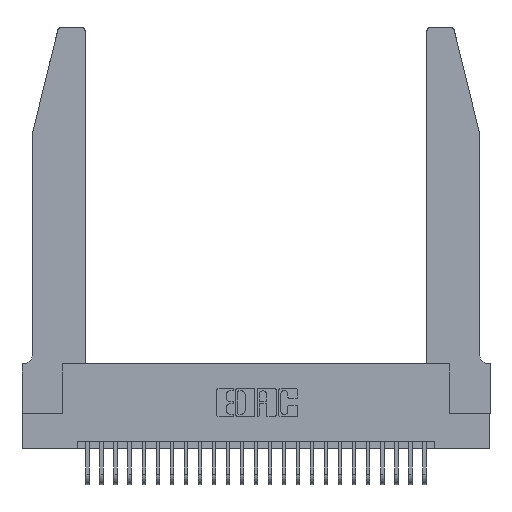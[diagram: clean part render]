
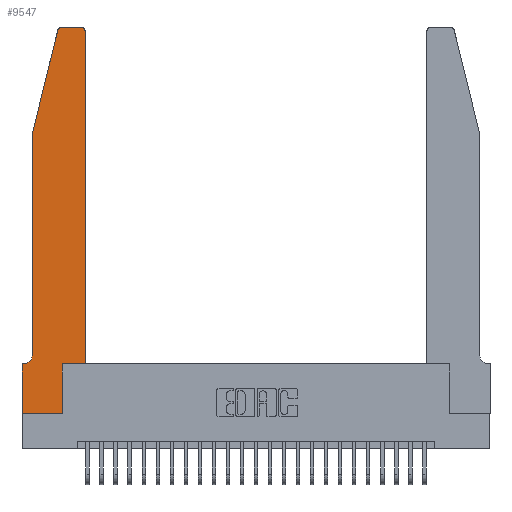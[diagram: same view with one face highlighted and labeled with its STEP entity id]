
A CAD part, top view. The second image highlights one B-rep face of the part: STEP entity #9547.
In plain terms, the highlighted planar face has unit normal (0, 0, 1).
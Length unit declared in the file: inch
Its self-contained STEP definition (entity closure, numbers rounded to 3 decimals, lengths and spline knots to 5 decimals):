
#465 = LINE ( 'NONE', #25406, #22419 ) ;
#1159 = PLANE ( 'NONE',  #19216 ) ;
#1476 = VECTOR ( 'NONE', #2208, 39.37008 ) ;
#1541 = CIRCLE ( 'NONE', #20087, 0.07 ) ;
#1642 = VERTEX_POINT ( 'NONE', #18377 ) ;
#1808 = CARTESIAN_POINT ( 'NONE',  ( 0.4505, 0.35, 0.37 ) ) ;
#1850 = ORIENTED_EDGE ( 'NONE', *, *, #24997, .T. ) ;
#2022 = EDGE_CURVE ( 'NONE', #19401, #26166, #21183, .T. ) ;
#2190 = CARTESIAN_POINT ( 'NONE',  ( 0.0755, 2., 0.37 ) ) ;
#2208 = DIRECTION ( 'NONE',  ( 0., -1., 0. ) ) ;
#2217 = EDGE_LOOP ( 'NONE', ( #2348, #25640, #6581, #22094, #24054, #10860, #9317, #10943, #26642, #17401, #20785, #1850 ) ) ;
#2271 = EDGE_CURVE ( 'NONE', #21834, #15559, #9877, .T. ) ;
#2348 = ORIENTED_EDGE ( 'NONE', *, *, #2634, .T. ) ;
#2413 = CARTESIAN_POINT ( 'NONE',  ( 0.25487, 2.72718, 0.37 ) ) ;
#2634 = EDGE_CURVE ( 'NONE', #8302, #1642, #24844, .T. ) ;
#2862 = CARTESIAN_POINT ( 'NONE',  ( 0.4205, 2.75, 0.37 ) ) ;
#2946 = CARTESIAN_POINT ( 'NONE',  ( 0.0055, 0.35, 0.37 ) ) ;
#3016 = VERTEX_POINT ( 'NONE', #5302 ) ;
#3129 = CARTESIAN_POINT ( 'NONE',  ( 0.4205, 2.72, 0.37 ) ) ;
#3370 = DIRECTION ( 'NONE',  ( 1., 0., 0. ) ) ;
#4426 = DIRECTION ( 'NONE',  ( -0.239, -0.971, 0. ) ) ;
#5302 = CARTESIAN_POINT ( 'NONE',  ( 0.4505, 2.72, 0.37 ) ) ;
#5370 = DIRECTION ( 'NONE',  ( 1., 0., 0. ) ) ;
#5846 = AXIS2_PLACEMENT_3D ( 'NONE', #11664, #26848, #13917 ) ;
#6477 = LINE ( 'NONE', #13195, #23227 ) ;
#6581 = ORIENTED_EDGE ( 'NONE', *, *, #9818, .T. ) ;
#6863 = VERTEX_POINT ( 'NONE', #2413 ) ;
#7178 = CARTESIAN_POINT ( 'NONE',  ( 0.0755, 2., 0.37 ) ) ;
#7501 = VECTOR ( 'NONE', #8138, 39.37008 ) ;
#8138 = DIRECTION ( 'NONE',  ( 1., 0., 0. ) ) ;
#8302 = VERTEX_POINT ( 'NONE', #2862 ) ;
#8848 = VECTOR ( 'NONE', #10862, 39.37008 ) ;
#8885 = DIRECTION ( 'NONE',  ( -1., 0., 0. ) ) ;
#9123 = CARTESIAN_POINT ( 'NONE',  ( 0.0055, 0.42, 0.37 ) ) ;
#9317 = ORIENTED_EDGE ( 'NONE', *, *, #11057, .T. ) ;
#9547 = ADVANCED_FACE ( 'NONE', ( #15391 ), #1159, .T. ) ;
#9818 = EDGE_CURVE ( 'NONE', #6863, #21834, #20143, .T. ) ;
#9849 = CARTESIAN_POINT ( 'NONE',  ( 0.2865, 0.35, 0.37 ) ) ;
#9877 = LINE ( 'NONE', #7178, #25870 ) ;
#10860 = ORIENTED_EDGE ( 'NONE', *, *, #11080, .T. ) ;
#10862 = DIRECTION ( 'NONE',  ( 0., 1., 0. ) ) ;
#10899 = CARTESIAN_POINT ( 'NONE',  ( 0.0755, 2., 0.37 ) ) ;
#10943 = ORIENTED_EDGE ( 'NONE', *, *, #13175, .T. ) ;
#11057 = EDGE_CURVE ( 'NONE', #18265, #21191, #13936, .T. ) ;
#11080 = EDGE_CURVE ( 'NONE', #24962, #18265, #19053, .T. ) ;
#11344 = DIRECTION ( 'NONE',  ( -1., 0., 0. ) ) ;
#11621 = VERTEX_POINT ( 'NONE', #1808 ) ;
#11664 = CARTESIAN_POINT ( 'NONE',  ( 0.284, 2.72, 0.37 ) ) ;
#12181 = CARTESIAN_POINT ( 'NONE',  ( 0., 0.35, 0.37 ) ) ;
#12538 = VECTOR ( 'NONE', #8885, 39.37008 ) ;
#13175 = EDGE_CURVE ( 'NONE', #21191, #19401, #465, .T. ) ;
#13195 = CARTESIAN_POINT ( 'NONE',  ( 0.4505, 0.35, 0.37 ) ) ;
#13917 = DIRECTION ( 'NONE',  ( 1., 0., 0. ) ) ;
#13936 = LINE ( 'NONE', #19848, #1476 ) ;
#14284 = AXIS2_PLACEMENT_3D ( 'NONE', #3129, #18554, #5370 ) ;
#14348 = VECTOR ( 'NONE', #4426, 39.37008 ) ;
#15391 = FACE_OUTER_BOUND ( 'NONE', #2217, .T. ) ;
#15410 = DIRECTION ( 'NONE',  ( 0., 1., 0. ) ) ;
#15559 = VERTEX_POINT ( 'NONE', #16978 ) ;
#16593 = DIRECTION ( 'NONE',  ( 0., 0., 1. ) ) ;
#16822 = DIRECTION ( 'NONE',  ( 1., 0., 0. ) ) ;
#16978 = CARTESIAN_POINT ( 'NONE',  ( 0.0755, 0.42, 0.37 ) ) ;
#17401 = ORIENTED_EDGE ( 'NONE', *, *, #17478, .T. ) ;
#17478 = EDGE_CURVE ( 'NONE', #26166, #11621, #22882, .T. ) ;
#17486 = CARTESIAN_POINT ( 'NONE',  ( 0.2865, 0.35, 0.37 ) ) ;
#17915 = CIRCLE ( 'NONE', #5846, 0.03 ) ;
#18265 = VERTEX_POINT ( 'NONE', #25916 ) ;
#18377 = CARTESIAN_POINT ( 'NONE',  ( 0.284, 2.75, 0.37 ) ) ;
#18554 = DIRECTION ( 'NONE',  ( 0., 0., 1. ) ) ;
#19053 = LINE ( 'NONE', #21982, #12538 ) ;
#19216 = AXIS2_PLACEMENT_3D ( 'NONE', #12181, #16593, #3370 ) ;
#19279 = CARTESIAN_POINT ( 'NONE',  ( 0.2605, 2.75, 0.37 ) ) ;
#19401 = VERTEX_POINT ( 'NONE', #27067 ) ;
#19848 = CARTESIAN_POINT ( 'NONE',  ( 0., 0., 0.37 ) ) ;
#19919 = EDGE_CURVE ( 'NONE', #1642, #6863, #17915, .T. ) ;
#20087 = AXIS2_PLACEMENT_3D ( 'NONE', #9123, #24378, #11344 ) ;
#20143 = LINE ( 'NONE', #2190, #14348 ) ;
#20785 = ORIENTED_EDGE ( 'NONE', *, *, #20881, .T. ) ;
#20881 = EDGE_CURVE ( 'NONE', #11621, #3016, #6477, .T. ) ;
#21183 = LINE ( 'NONE', #17486, #8848 ) ;
#21191 = VERTEX_POINT ( 'NONE', #27163 ) ;
#21260 = CARTESIAN_POINT ( 'NONE',  ( 0.4505, 0.35, 0.37 ) ) ;
#21431 = DIRECTION ( 'NONE',  ( -1., 0., 0. ) ) ;
#21834 = VERTEX_POINT ( 'NONE', #10899 ) ;
#21982 = CARTESIAN_POINT ( 'NONE',  ( 0.0755, 0.35, 0.37 ) ) ;
#22094 = ORIENTED_EDGE ( 'NONE', *, *, #2271, .T. ) ;
#22419 = VECTOR ( 'NONE', #16822, 39.37008 ) ;
#22430 = EDGE_CURVE ( 'NONE', #15559, #24962, #1541, .T. ) ;
#22882 = LINE ( 'NONE', #21260, #7501 ) ;
#22985 = CIRCLE ( 'NONE', #14284, 0.03 ) ;
#23227 = VECTOR ( 'NONE', #15410, 39.37008 ) ;
#23504 = VECTOR ( 'NONE', #21431, 39.37008 ) ;
#24054 = ORIENTED_EDGE ( 'NONE', *, *, #22430, .T. ) ;
#24378 = DIRECTION ( 'NONE',  ( 0., 0., -1. ) ) ;
#24844 = LINE ( 'NONE', #19279, #23504 ) ;
#24962 = VERTEX_POINT ( 'NONE', #2946 ) ;
#24997 = EDGE_CURVE ( 'NONE', #3016, #8302, #22985, .T. ) ;
#25406 = CARTESIAN_POINT ( 'NONE',  ( 0., 0., 0.37 ) ) ;
#25640 = ORIENTED_EDGE ( 'NONE', *, *, #19919, .T. ) ;
#25870 = VECTOR ( 'NONE', #26699, 39.37008 ) ;
#25916 = CARTESIAN_POINT ( 'NONE',  ( 0., 0.35, 0.37 ) ) ;
#26166 = VERTEX_POINT ( 'NONE', #9849 ) ;
#26642 = ORIENTED_EDGE ( 'NONE', *, *, #2022, .T. ) ;
#26699 = DIRECTION ( 'NONE',  ( 0., -1., 0. ) ) ;
#26848 = DIRECTION ( 'NONE',  ( 0., 0., 1. ) ) ;
#27067 = CARTESIAN_POINT ( 'NONE',  ( 0.2865, 0., 0.37 ) ) ;
#27163 = CARTESIAN_POINT ( 'NONE',  ( 0., 0., 0.37 ) ) ;
